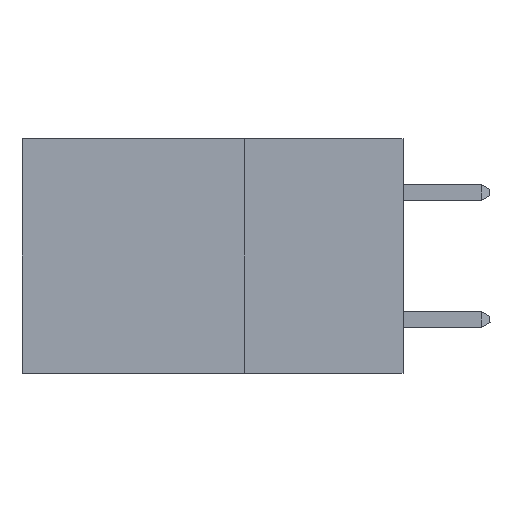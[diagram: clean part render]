
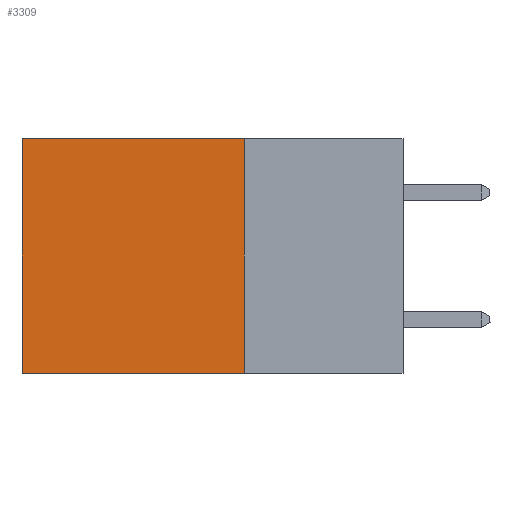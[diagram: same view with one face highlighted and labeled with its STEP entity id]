
A CAD part, left-side view. The second image highlights one B-rep face of the part: STEP entity #3309.
In plain terms, the highlighted planar face has unit normal (-1, 0, 0).
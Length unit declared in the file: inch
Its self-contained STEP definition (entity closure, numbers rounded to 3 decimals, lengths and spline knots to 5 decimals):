
#301 = CARTESIAN_POINT ( 'NONE',  ( 0.2875, 0.25, -0.37 ) ) ;
#1259 = VERTEX_POINT ( 'NONE', #4964 ) ;
#2602 = EDGE_CURVE ( 'NONE', #15127, #1259, #15379, .T. ) ;
#3309 = ADVANCED_FACE ( 'NONE', ( #8940 ), #18729, .F. ) ;
#3400 = DIRECTION ( 'NONE',  ( 0., 0., -1. ) ) ;
#3949 = VECTOR ( 'NONE', #23138, 39.37008 ) ;
#4964 = CARTESIAN_POINT ( 'NONE',  ( 0.2875, 0.6, 0. ) ) ;
#5368 = LINE ( 'NONE', #26581, #27642 ) ;
#5373 = EDGE_LOOP ( 'NONE', ( #27240, #19811, #12249, #22327 ) ) ;
#5574 = LINE ( 'NONE', #301, #7238 ) ;
#7238 = VECTOR ( 'NONE', #25687, 39.37008 ) ;
#7378 = CARTESIAN_POINT ( 'NONE',  ( 0.2875, 0.25, -0.37 ) ) ;
#8128 = CARTESIAN_POINT ( 'NONE',  ( 0.2875, 0.6, -0.37 ) ) ;
#8940 = FACE_OUTER_BOUND ( 'NONE', #5373, .T. ) ;
#9892 = EDGE_CURVE ( 'NONE', #15127, #17468, #11771, .T. ) ;
#10088 = CARTESIAN_POINT ( 'NONE',  ( 0.2875, 0.25, 0. ) ) ;
#10110 = VERTEX_POINT ( 'NONE', #8128 ) ;
#10444 = VECTOR ( 'NONE', #24140, 39.37008 ) ;
#11771 = LINE ( 'NONE', #19872, #10444 ) ;
#12249 = ORIENTED_EDGE ( 'NONE', *, *, #9892, .F. ) ;
#13033 = EDGE_CURVE ( 'NONE', #17468, #10110, #5574, .T. ) ;
#15127 = VERTEX_POINT ( 'NONE', #18517 ) ;
#15379 = LINE ( 'NONE', #10088, #3949 ) ;
#16365 = DIRECTION ( 'NONE',  ( 1., 0., 0. ) ) ;
#17468 = VERTEX_POINT ( 'NONE', #7378 ) ;
#18503 = AXIS2_PLACEMENT_3D ( 'NONE', #20449, #16365, #3400 ) ;
#18517 = CARTESIAN_POINT ( 'NONE',  ( 0.2875, 0.25, 0. ) ) ;
#18729 = PLANE ( 'NONE',  #18503 ) ;
#19811 = ORIENTED_EDGE ( 'NONE', *, *, #13033, .F. ) ;
#19872 = CARTESIAN_POINT ( 'NONE',  ( 0.2875, 0.25, 0. ) ) ;
#20340 = DIRECTION ( 'NONE',  ( 0., 0., -1. ) ) ;
#20449 = CARTESIAN_POINT ( 'NONE',  ( 0.2875, 0.25, 0. ) ) ;
#22327 = ORIENTED_EDGE ( 'NONE', *, *, #2602, .T. ) ;
#23138 = DIRECTION ( 'NONE',  ( 0., 1., 0. ) ) ;
#24140 = DIRECTION ( 'NONE',  ( 0., 0., -1. ) ) ;
#24208 = EDGE_CURVE ( 'NONE', #1259, #10110, #5368, .T. ) ;
#25687 = DIRECTION ( 'NONE',  ( 0., 1., 0. ) ) ;
#26581 = CARTESIAN_POINT ( 'NONE',  ( 0.2875, 0.6, 0. ) ) ;
#27240 = ORIENTED_EDGE ( 'NONE', *, *, #24208, .T. ) ;
#27642 = VECTOR ( 'NONE', #20340, 39.37008 ) ;
